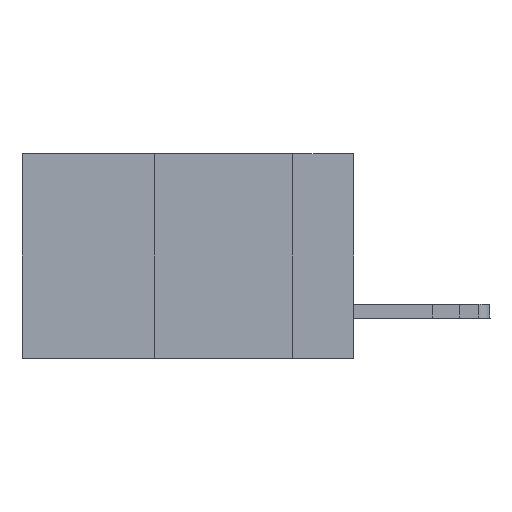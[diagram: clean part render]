
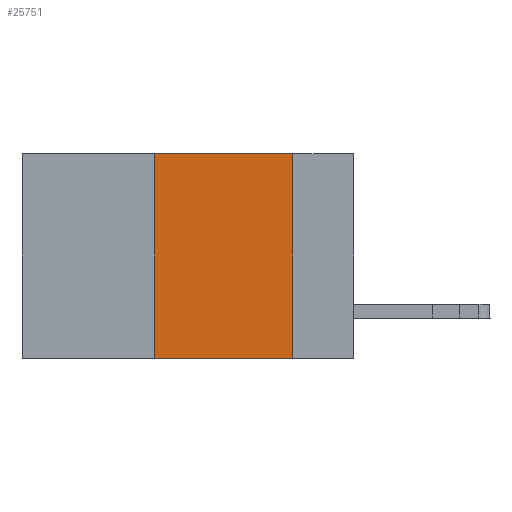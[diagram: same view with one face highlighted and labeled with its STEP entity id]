
A CAD part, left-side view. The second image highlights one B-rep face of the part: STEP entity #25751.
In plain terms, the highlighted planar face has unit normal (-1, 0, 0).
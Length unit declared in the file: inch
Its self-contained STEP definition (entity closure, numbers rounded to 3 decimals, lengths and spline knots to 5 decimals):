
#1071 = DIRECTION ( 'NONE',  ( 0., -1., 0. ) ) ;
#1150 = VERTEX_POINT ( 'NONE', #26740 ) ;
#1434 = CARTESIAN_POINT ( 'NONE',  ( 0., 0.11, 0. ) ) ;
#1462 = CARTESIAN_POINT ( 'NONE',  ( 0., 0.36, 0. ) ) ;
#1593 = LINE ( 'NONE', #9468, #8821 ) ;
#1660 = VECTOR ( 'NONE', #21292, 39.37008 ) ;
#2605 = FACE_OUTER_BOUND ( 'NONE', #7656, .T. ) ;
#2742 = DIRECTION ( 'NONE',  ( 0., 0., 1. ) ) ;
#4037 = EDGE_CURVE ( 'NONE', #18240, #31205, #20360, .T. ) ;
#4962 = ORIENTED_EDGE ( 'NONE', *, *, #7269, .F. ) ;
#5339 = VECTOR ( 'NONE', #11703, 39.37008 ) ;
#7269 = EDGE_CURVE ( 'NONE', #1150, #31205, #28302, .T. ) ;
#7340 = LINE ( 'NONE', #8624, #30681 ) ;
#7656 = EDGE_LOOP ( 'NONE', ( #4962, #18551, #27327, #18289 ) ) ;
#8404 = AXIS2_PLACEMENT_3D ( 'NONE', #22372, #19671, #12346 ) ;
#8624 = CARTESIAN_POINT ( 'NONE',  ( 0., 0.6, 0. ) ) ;
#8821 = VECTOR ( 'NONE', #2742, 39.37008 ) ;
#9468 = CARTESIAN_POINT ( 'NONE',  ( 0., 0.36, 0. ) ) ;
#11400 = CARTESIAN_POINT ( 'NONE',  ( 0., 0.11, -0.37 ) ) ;
#11703 = DIRECTION ( 'NONE',  ( 0., 0., -1. ) ) ;
#11794 = EDGE_CURVE ( 'NONE', #29102, #1150, #7340, .T. ) ;
#12346 = DIRECTION ( 'NONE',  ( 0., 0., -1. ) ) ;
#12870 = EDGE_CURVE ( 'NONE', #18240, #29102, #1593, .T. ) ;
#16651 = CARTESIAN_POINT ( 'NONE',  ( 0., 0.6, -0.37 ) ) ;
#18138 = CARTESIAN_POINT ( 'NONE',  ( 0., 0.36, -0.37 ) ) ;
#18240 = VERTEX_POINT ( 'NONE', #18138 ) ;
#18289 = ORIENTED_EDGE ( 'NONE', *, *, #4037, .T. ) ;
#18551 = ORIENTED_EDGE ( 'NONE', *, *, #11794, .F. ) ;
#19671 = DIRECTION ( 'NONE',  ( 1., 0., 0. ) ) ;
#19986 = PLANE ( 'NONE',  #8404 ) ;
#20360 = LINE ( 'NONE', #16651, #1660 ) ;
#21292 = DIRECTION ( 'NONE',  ( 0., -1., 0. ) ) ;
#22372 = CARTESIAN_POINT ( 'NONE',  ( 0., 0.6, 0. ) ) ;
#25751 = ADVANCED_FACE ( 'NONE', ( #2605 ), #19986, .F. ) ;
#26740 = CARTESIAN_POINT ( 'NONE',  ( 0., 0.11, 0. ) ) ;
#27327 = ORIENTED_EDGE ( 'NONE', *, *, #12870, .F. ) ;
#28302 = LINE ( 'NONE', #1434, #5339 ) ;
#29102 = VERTEX_POINT ( 'NONE', #1462 ) ;
#30681 = VECTOR ( 'NONE', #1071, 39.37008 ) ;
#31205 = VERTEX_POINT ( 'NONE', #11400 ) ;
